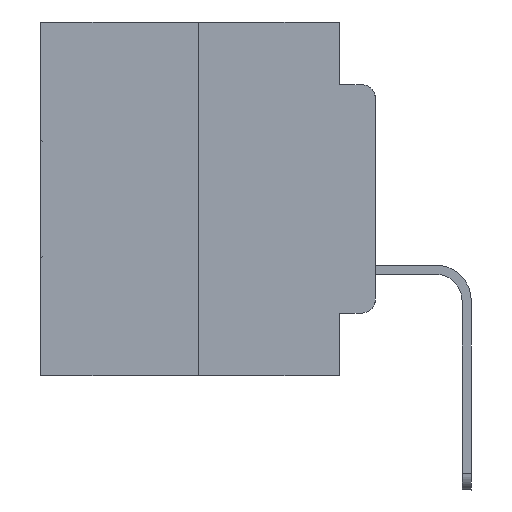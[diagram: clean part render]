
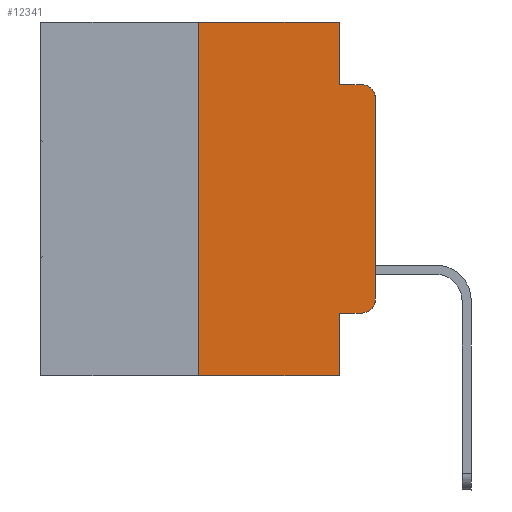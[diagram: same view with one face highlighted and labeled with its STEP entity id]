
A CAD part, left-side view. The second image highlights one B-rep face of the part: STEP entity #12341.
In plain terms, the highlighted planar face has unit normal (-1, 0, 0).
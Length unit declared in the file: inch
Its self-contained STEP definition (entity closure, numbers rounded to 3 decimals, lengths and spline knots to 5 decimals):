
#526 = ORIENTED_EDGE ( 'NONE', *, *, #8740, .F. ) ;
#556 = CARTESIAN_POINT ( 'NONE',  ( 0., 0.473, 0. ) ) ;
#647 = DIRECTION ( 'NONE',  ( 0., -1., 0. ) ) ;
#1196 = DIRECTION ( 'NONE',  ( 0., 0., -1. ) ) ;
#1295 = DIRECTION ( 'NONE',  ( 0., 0., 1. ) ) ;
#2129 = CARTESIAN_POINT ( 'NONE',  ( 0., 0.02, -0.1085 ) ) ;
#2227 = DIRECTION ( 'NONE',  ( 1., 0., 0. ) ) ;
#2335 = ORIENTED_EDGE ( 'NONE', *, *, #17846, .T. ) ;
#2510 = DIRECTION ( 'NONE',  ( 0., -1., 0. ) ) ;
#2801 = VERTEX_POINT ( 'NONE', #13901 ) ;
#3588 = CARTESIAN_POINT ( 'NONE',  ( 0., 0.051, 0. ) ) ;
#3864 = DIRECTION ( 'NONE',  ( 0., -1., 0. ) ) ;
#4012 = CARTESIAN_POINT ( 'NONE',  ( 0., 0.051, -0.0885 ) ) ;
#4118 = DIRECTION ( 'NONE',  ( 0., -1., 0. ) ) ;
#4217 = DIRECTION ( 'NONE',  ( -1., 0., 0. ) ) ;
#5192 = CARTESIAN_POINT ( 'NONE',  ( 0., 0.051, -0.0885 ) ) ;
#5736 = CARTESIAN_POINT ( 'NONE',  ( 0., 0.25, 0. ) ) ;
#5944 = AXIS2_PLACEMENT_3D ( 'NONE', #2129, #4217, #28965 ) ;
#6449 = CARTESIAN_POINT ( 'NONE',  ( 0., 0.051, 0. ) ) ;
#6958 = ORIENTED_EDGE ( 'NONE', *, *, #8831, .T. ) ;
#7475 = CARTESIAN_POINT ( 'NONE',  ( 0., 0.25, 0. ) ) ;
#7844 = VECTOR ( 'NONE', #2510, 39.37008 ) ;
#8216 = ORIENTED_EDGE ( 'NONE', *, *, #9740, .F. ) ;
#8220 = LINE ( 'NONE', #15752, #7844 ) ;
#8740 = EDGE_CURVE ( 'NONE', #20676, #19396, #28562, .T. ) ;
#8831 = EDGE_CURVE ( 'NONE', #12598, #21673, #16899, .T. ) ;
#8949 = PLANE ( 'NONE',  #20200 ) ;
#9740 = EDGE_CURVE ( 'NONE', #19396, #12655, #14745, .T. ) ;
#10042 = CARTESIAN_POINT ( 'NONE',  ( 0., 0.473, 0. ) ) ;
#10179 = CARTESIAN_POINT ( 'NONE',  ( 0., 0.051, 0. ) ) ;
#10306 = DIRECTION ( 'NONE',  ( 0., 0., -1. ) ) ;
#10649 = VERTEX_POINT ( 'NONE', #5192 ) ;
#10917 = VECTOR ( 'NONE', #14653, 39.37008 ) ;
#10941 = ORIENTED_EDGE ( 'NONE', *, *, #23847, .T. ) ;
#10959 = LINE ( 'NONE', #4012, #27158 ) ;
#11076 = ORIENTED_EDGE ( 'NONE', *, *, #19752, .F. ) ;
#11487 = CARTESIAN_POINT ( 'NONE',  ( 0., 0.02, -0.4115 ) ) ;
#12286 = EDGE_CURVE ( 'NONE', #20676, #26805, #8220, .T. ) ;
#12341 = ADVANCED_FACE ( 'NONE', ( #14919 ), #8949, .F. ) ;
#12598 = VERTEX_POINT ( 'NONE', #17036 ) ;
#12643 = DIRECTION ( 'NONE',  ( -1., 0., 0. ) ) ;
#12655 = VERTEX_POINT ( 'NONE', #6449 ) ;
#13642 = ORIENTED_EDGE ( 'NONE', *, *, #20912, .F. ) ;
#13901 = CARTESIAN_POINT ( 'NONE',  ( 0., 0., -0.1085 ) ) ;
#14373 = VECTOR ( 'NONE', #28794, 39.37008 ) ;
#14653 = DIRECTION ( 'NONE',  ( 0., 0., 1. ) ) ;
#14745 = LINE ( 'NONE', #556, #19342 ) ;
#14752 = CARTESIAN_POINT ( 'NONE',  ( 0., 0.02, -0.0885 ) ) ;
#14827 = EDGE_CURVE ( 'NONE', #12598, #26805, #22213, .T. ) ;
#14919 = FACE_OUTER_BOUND ( 'NONE', #16868, .T. ) ;
#15752 = CARTESIAN_POINT ( 'NONE',  ( 0., 0.473, -0.5 ) ) ;
#15937 = DIRECTION ( 'NONE',  ( 0., 0., -1. ) ) ;
#16160 = LINE ( 'NONE', #10179, #14373 ) ;
#16868 = EDGE_LOOP ( 'NONE', ( #21893, #2335, #11076, #13642, #8216, #526, #20057, #22169, #6958, #10941 ) ) ;
#16899 = LINE ( 'NONE', #26341, #26433 ) ;
#17036 = CARTESIAN_POINT ( 'NONE',  ( 0., 0.051, -0.4115 ) ) ;
#17276 = VECTOR ( 'NONE', #1295, 39.37008 ) ;
#17846 = EDGE_CURVE ( 'NONE', #2801, #26735, #27632, .T. ) ;
#18740 = CARTESIAN_POINT ( 'NONE',  ( 0., 0.25, -0.5 ) ) ;
#19342 = VECTOR ( 'NONE', #647, 39.37008 ) ;
#19396 = VERTEX_POINT ( 'NONE', #7475 ) ;
#19411 = CARTESIAN_POINT ( 'NONE',  ( 0., 0., 0. ) ) ;
#19752 = EDGE_CURVE ( 'NONE', #10649, #26735, #10959, .T. ) ;
#20057 = ORIENTED_EDGE ( 'NONE', *, *, #12286, .T. ) ;
#20200 = AXIS2_PLACEMENT_3D ( 'NONE', #10042, #2227, #15937 ) ;
#20450 = VECTOR ( 'NONE', #10306, 39.37008 ) ;
#20676 = VERTEX_POINT ( 'NONE', #18740 ) ;
#20791 = CARTESIAN_POINT ( 'NONE',  ( 0., 0., -0.3915 ) ) ;
#20912 = EDGE_CURVE ( 'NONE', #12655, #10649, #16160, .T. ) ;
#21625 = CARTESIAN_POINT ( 'NONE',  ( 0., 0.02, -0.3915 ) ) ;
#21673 = VERTEX_POINT ( 'NONE', #11487 ) ;
#21893 = ORIENTED_EDGE ( 'NONE', *, *, #26750, .T. ) ;
#22169 = ORIENTED_EDGE ( 'NONE', *, *, #14827, .F. ) ;
#22213 = LINE ( 'NONE', #3588, #20450 ) ;
#22219 = LINE ( 'NONE', #19411, #10917 ) ;
#22700 = AXIS2_PLACEMENT_3D ( 'NONE', #21625, #12643, #1196 ) ;
#23069 = CIRCLE ( 'NONE', #22700, 0.02 ) ;
#23847 = EDGE_CURVE ( 'NONE', #21673, #24858, #23069, .T. ) ;
#24858 = VERTEX_POINT ( 'NONE', #20791 ) ;
#26341 = CARTESIAN_POINT ( 'NONE',  ( 0., 0.051, -0.4115 ) ) ;
#26433 = VECTOR ( 'NONE', #3864, 39.37008 ) ;
#26735 = VERTEX_POINT ( 'NONE', #14752 ) ;
#26750 = EDGE_CURVE ( 'NONE', #24858, #2801, #22219, .T. ) ;
#26805 = VERTEX_POINT ( 'NONE', #28749 ) ;
#27158 = VECTOR ( 'NONE', #4118, 39.37008 ) ;
#27632 = CIRCLE ( 'NONE', #5944, 0.02 ) ;
#28562 = LINE ( 'NONE', #5736, #17276 ) ;
#28749 = CARTESIAN_POINT ( 'NONE',  ( 0., 0.051, -0.5 ) ) ;
#28794 = DIRECTION ( 'NONE',  ( 0., 0., -1. ) ) ;
#28965 = DIRECTION ( 'NONE',  ( 0., 0., -1. ) ) ;
